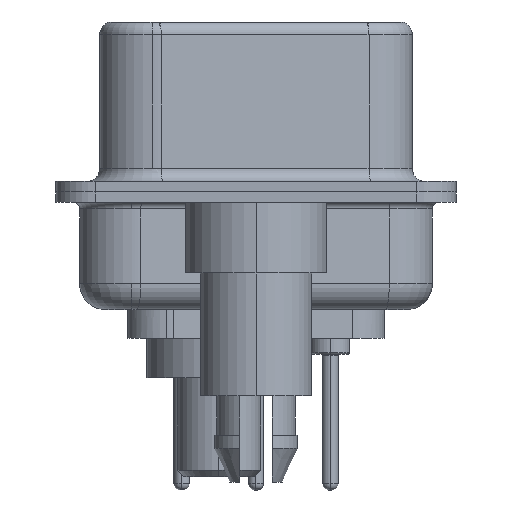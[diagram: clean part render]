
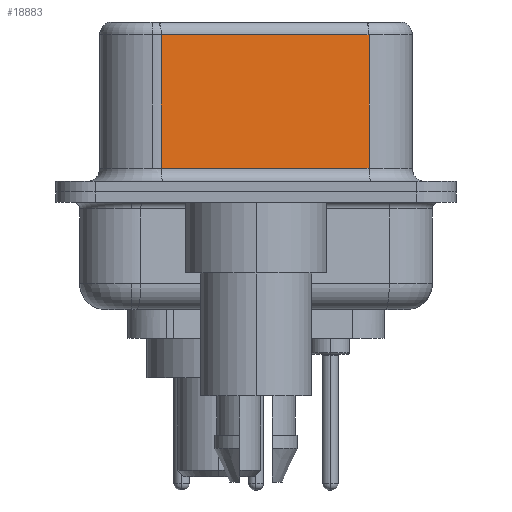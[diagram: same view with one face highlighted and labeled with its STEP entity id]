
A CAD part, left-side view. The second image highlights one B-rep face of the part: STEP entity #18883.
In plain terms, the highlighted planar face has unit normal (-0.985, -0.174, 0).
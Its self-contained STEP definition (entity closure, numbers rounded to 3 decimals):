
#1902 = CARTESIAN_POINT ( 'NONE',  ( 3.73, 3.628, 6.52 ) ) ;
#2660 = ORIENTED_EDGE ( 'NONE', *, *, #24270, .T. ) ;
#2994 = DIRECTION ( 'NONE',  ( 0.174, -0.985, 0. ) ) ;
#3732 = EDGE_CURVE ( 'NONE', #3752, #19145, #8426, .T. ) ;
#3752 = VERTEX_POINT ( 'NONE', #7722 ) ;
#4299 = LINE ( 'NONE', #9980, #9376 ) ;
#4849 = EDGE_LOOP ( 'NONE', ( #8348, #12243, #2660, #7410 ) ) ;
#5004 = FACE_OUTER_BOUND ( 'NONE', #4849, .T. ) ;
#5032 = EDGE_CURVE ( 'NONE', #18437, #17806, #23782, .T. ) ;
#7175 = CARTESIAN_POINT ( 'NONE',  ( 5.132, -4.322, 0.9 ) ) ;
#7410 = ORIENTED_EDGE ( 'NONE', *, *, #3732, .T. ) ;
#7722 = CARTESIAN_POINT ( 'NONE',  ( 3.73, 3.628, 0.9 ) ) ;
#7787 = EDGE_CURVE ( 'NONE', #18437, #19145, #4299, .T. ) ;
#8348 = ORIENTED_EDGE ( 'NONE', *, *, #7787, .F. ) ;
#8426 = LINE ( 'NONE', #7175, #26860 ) ;
#9376 = VECTOR ( 'NONE', #18119, 1000. ) ;
#9496 = CARTESIAN_POINT ( 'NONE',  ( 5.132, -4.322, 6.52 ) ) ;
#9980 = CARTESIAN_POINT ( 'NONE',  ( 5.132, -4.322, 6.52 ) ) ;
#10226 = DIRECTION ( 'NONE',  ( -0.174, 0.985, 0. ) ) ;
#12243 = ORIENTED_EDGE ( 'NONE', *, *, #5032, .T. ) ;
#13288 = VECTOR ( 'NONE', #10226, 1000. ) ;
#14337 = PLANE ( 'NONE',  #17128 ) ;
#14451 = DIRECTION ( 'NONE',  ( 0.985, 0.174, 0. ) ) ;
#16453 = VECTOR ( 'NONE', #18965, 1000. ) ;
#17128 = AXIS2_PLACEMENT_3D ( 'NONE', #9496, #14451, #31145 ) ;
#17552 = CARTESIAN_POINT ( 'NONE',  ( 5.132, -4.322, 6.02 ) ) ;
#17806 = VERTEX_POINT ( 'NONE', #22138 ) ;
#17810 = CARTESIAN_POINT ( 'NONE',  ( 5.132, -4.322, 0.9 ) ) ;
#18119 = DIRECTION ( 'NONE',  ( 0., 0., -1. ) ) ;
#18437 = VERTEX_POINT ( 'NONE', #17552 ) ;
#18883 = ADVANCED_FACE ( 'NONE', ( #5004 ), #14337, .F. ) ;
#18965 = DIRECTION ( 'NONE',  ( 0., 0., -1. ) ) ;
#19145 = VERTEX_POINT ( 'NONE', #17810 ) ;
#22025 = LINE ( 'NONE', #1902, #16453 ) ;
#22138 = CARTESIAN_POINT ( 'NONE',  ( 3.73, 3.628, 6.02 ) ) ;
#23782 = LINE ( 'NONE', #24294, #13288 ) ;
#24270 = EDGE_CURVE ( 'NONE', #17806, #3752, #22025, .T. ) ;
#24294 = CARTESIAN_POINT ( 'NONE',  ( 5.132, -4.322, 6.02 ) ) ;
#26860 = VECTOR ( 'NONE', #2994, 1000. ) ;
#31145 = DIRECTION ( 'NONE',  ( -0.174, 0.985, 0. ) ) ;
